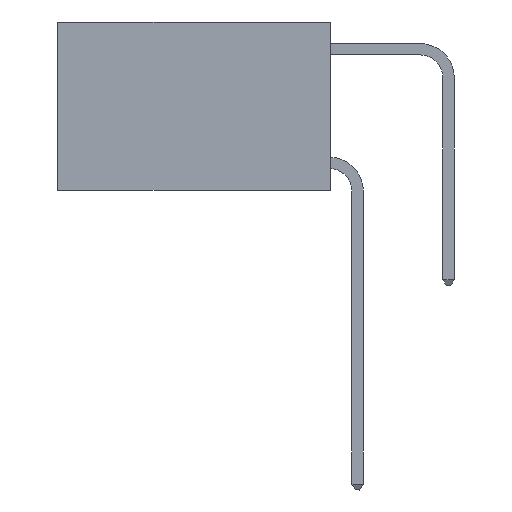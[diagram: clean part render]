
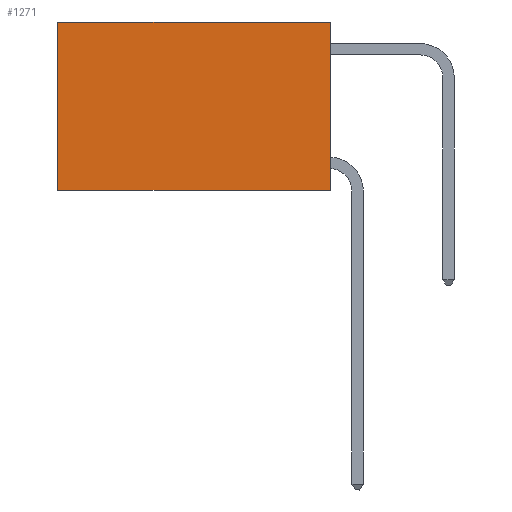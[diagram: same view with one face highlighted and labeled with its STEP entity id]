
A CAD part, left-side view. The second image highlights one B-rep face of the part: STEP entity #1271.
In plain terms, the highlighted planar face has unit normal (-1, 0, 0).
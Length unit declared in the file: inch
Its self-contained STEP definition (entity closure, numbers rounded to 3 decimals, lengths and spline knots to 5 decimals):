
#481 = ORIENTED_EDGE ( 'NONE', *, *, #8054, .T. ) ;
#562 = AXIS2_PLACEMENT_3D ( 'NONE', #6136, #7348, #3196 ) ;
#642 = LINE ( 'NONE', #5408, #5117 ) ;
#1271 = ADVANCED_FACE ( 'NONE', ( #6398 ), #1785, .F. ) ;
#1349 = CARTESIAN_POINT ( 'NONE',  ( 0.2625, 0.6, 0. ) ) ;
#1605 = EDGE_CURVE ( 'NONE', #5143, #1904, #4818, .T. ) ;
#1785 = PLANE ( 'NONE',  #562 ) ;
#1904 = VERTEX_POINT ( 'NONE', #6284 ) ;
#2097 = CARTESIAN_POINT ( 'NONE',  ( 0.2625, 0.6, 0. ) ) ;
#2286 = VECTOR ( 'NONE', #5701, 39.37008 ) ;
#2798 = VERTEX_POINT ( 'NONE', #8470 ) ;
#3196 = DIRECTION ( 'NONE',  ( 0., 0., -1. ) ) ;
#4642 = DIRECTION ( 'NONE',  ( 0., 1., 0. ) ) ;
#4658 = EDGE_LOOP ( 'NONE', ( #9018, #6545, #7642, #481 ) ) ;
#4818 = LINE ( 'NONE', #2097, #8045 ) ;
#4966 = CARTESIAN_POINT ( 'NONE',  ( 0.2625, 0., -0.37 ) ) ;
#5117 = VECTOR ( 'NONE', #4642, 39.37008 ) ;
#5143 = VERTEX_POINT ( 'NONE', #1349 ) ;
#5408 = CARTESIAN_POINT ( 'NONE',  ( 0.2625, 0., 0. ) ) ;
#5419 = VERTEX_POINT ( 'NONE', #7902 ) ;
#5701 = DIRECTION ( 'NONE',  ( 0., 1., 0. ) ) ;
#6136 = CARTESIAN_POINT ( 'NONE',  ( 0.2625, 0., 0. ) ) ;
#6284 = CARTESIAN_POINT ( 'NONE',  ( 0.2625, 0.6, -0.37 ) ) ;
#6398 = FACE_OUTER_BOUND ( 'NONE', #4658, .T. ) ;
#6429 = EDGE_CURVE ( 'NONE', #5419, #2798, #8639, .T. ) ;
#6451 = VECTOR ( 'NONE', #7923, 39.37008 ) ;
#6545 = ORIENTED_EDGE ( 'NONE', *, *, #9251, .F. ) ;
#7348 = DIRECTION ( 'NONE',  ( 1., 0., 0. ) ) ;
#7642 = ORIENTED_EDGE ( 'NONE', *, *, #6429, .F. ) ;
#7902 = CARTESIAN_POINT ( 'NONE',  ( 0.2625, 0., 0. ) ) ;
#7923 = DIRECTION ( 'NONE',  ( 0., 0., -1. ) ) ;
#7991 = DIRECTION ( 'NONE',  ( 0., 0., -1. ) ) ;
#8045 = VECTOR ( 'NONE', #7991, 39.37008 ) ;
#8054 = EDGE_CURVE ( 'NONE', #5419, #5143, #642, .T. ) ;
#8470 = CARTESIAN_POINT ( 'NONE',  ( 0.2625, 0., -0.37 ) ) ;
#8592 = LINE ( 'NONE', #4966, #2286 ) ;
#8639 = LINE ( 'NONE', #8649, #6451 ) ;
#8649 = CARTESIAN_POINT ( 'NONE',  ( 0.2625, 0., 0. ) ) ;
#9018 = ORIENTED_EDGE ( 'NONE', *, *, #1605, .T. ) ;
#9251 = EDGE_CURVE ( 'NONE', #2798, #1904, #8592, .T. ) ;
